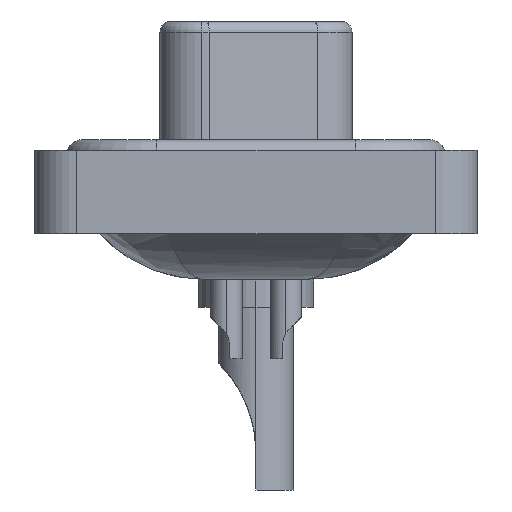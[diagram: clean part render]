
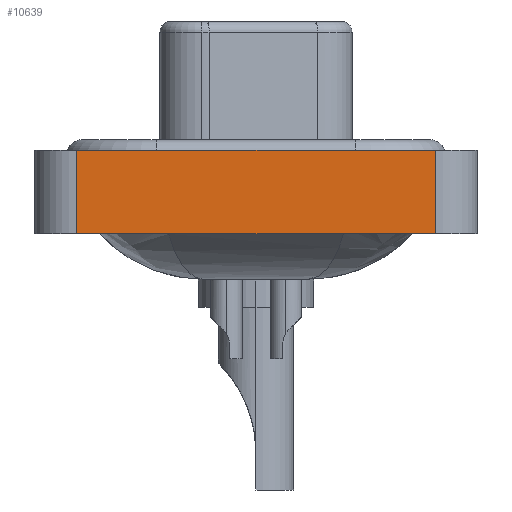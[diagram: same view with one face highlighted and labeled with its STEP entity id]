
A CAD part, left-side view. The second image highlights one B-rep face of the part: STEP entity #10639.
In plain terms, the highlighted planar face has unit normal (-1, 0, 0).
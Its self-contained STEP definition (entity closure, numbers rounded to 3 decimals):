
#1158 = CARTESIAN_POINT ( 'NONE',  ( -7.35, -8.55, 0.4 ) ) ;
#2299 = EDGE_LOOP ( 'NONE', ( #8470, #2688, #11127, #17902 ) ) ;
#2688 = ORIENTED_EDGE ( 'NONE', *, *, #7940, .F. ) ;
#3056 = CARTESIAN_POINT ( 'NONE',  ( -7.35, -8.55, -3.6 ) ) ;
#3389 = DIRECTION ( 'NONE',  ( 0., 0., 1. ) ) ;
#3857 = DIRECTION ( 'NONE',  ( 0., -1., 0. ) ) ;
#4049 = EDGE_CURVE ( 'NONE', #9685, #4857, #22706, .T. ) ;
#4857 = VERTEX_POINT ( 'NONE', #3056 ) ;
#5005 = CARTESIAN_POINT ( 'NONE',  ( -7.35, -8.55, 0.4 ) ) ;
#5510 = CARTESIAN_POINT ( 'NONE',  ( -7.35, -8.55, -3.6 ) ) ;
#5735 = CARTESIAN_POINT ( 'NONE',  ( -7.35, -8.55, -3.6 ) ) ;
#5782 = LINE ( 'NONE', #13562, #14170 ) ;
#6910 = LINE ( 'NONE', #5005, #13804 ) ;
#7940 = EDGE_CURVE ( 'NONE', #20100, #19157, #6910, .T. ) ;
#8470 = ORIENTED_EDGE ( 'NONE', *, *, #20894, .T. ) ;
#8865 = CARTESIAN_POINT ( 'NONE',  ( -7.35, 8.55, -3.6 ) ) ;
#8889 = DIRECTION ( 'NONE',  ( 0., -1., 0. ) ) ;
#8906 = PLANE ( 'NONE',  #23096 ) ;
#9685 = VERTEX_POINT ( 'NONE', #8865 ) ;
#10639 = ADVANCED_FACE ( 'NONE', ( #18313 ), #8906, .T. ) ;
#10791 = DIRECTION ( 'NONE',  ( 0., 0., 1. ) ) ;
#11066 = LINE ( 'NONE', #12951, #12070 ) ;
#11127 = ORIENTED_EDGE ( 'NONE', *, *, #17780, .F. ) ;
#12070 = VECTOR ( 'NONE', #3389, 1000. ) ;
#12951 = CARTESIAN_POINT ( 'NONE',  ( -7.35, 8.55, -3.6 ) ) ;
#13191 = DIRECTION ( 'NONE',  ( 0., 0., 1. ) ) ;
#13562 = CARTESIAN_POINT ( 'NONE',  ( -7.35, -8.55, -3.6 ) ) ;
#13804 = VECTOR ( 'NONE', #8889, 1000. ) ;
#14170 = VECTOR ( 'NONE', #13191, 1000. ) ;
#14426 = CARTESIAN_POINT ( 'NONE',  ( -7.35, 8.55, 0.4 ) ) ;
#17780 = EDGE_CURVE ( 'NONE', #9685, #20100, #11066, .T. ) ;
#17902 = ORIENTED_EDGE ( 'NONE', *, *, #4049, .T. ) ;
#18313 = FACE_OUTER_BOUND ( 'NONE', #2299, .T. ) ;
#19157 = VERTEX_POINT ( 'NONE', #1158 ) ;
#20100 = VERTEX_POINT ( 'NONE', #14426 ) ;
#20894 = EDGE_CURVE ( 'NONE', #4857, #19157, #5782, .T. ) ;
#20926 = DIRECTION ( 'NONE',  ( -1., 0., 0. ) ) ;
#22706 = LINE ( 'NONE', #5510, #23022 ) ;
#23022 = VECTOR ( 'NONE', #3857, 1000. ) ;
#23096 = AXIS2_PLACEMENT_3D ( 'NONE', #5735, #20926, #10791 ) ;
